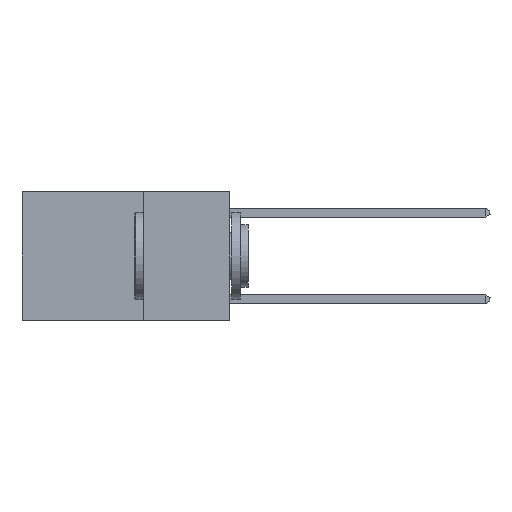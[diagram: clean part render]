
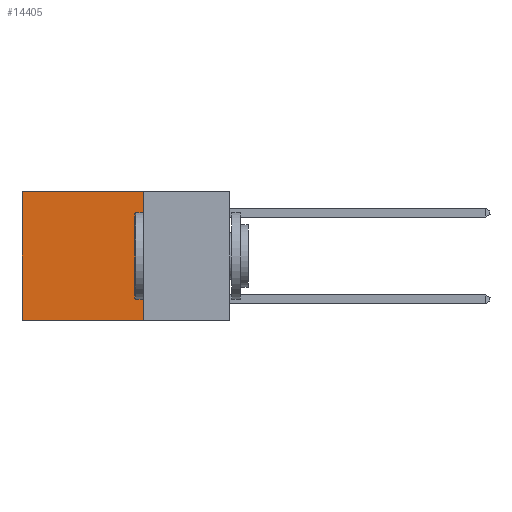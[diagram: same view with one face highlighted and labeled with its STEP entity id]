
A CAD part, left-side view. The second image highlights one B-rep face of the part: STEP entity #14405.
In plain terms, the highlighted planar face has unit normal (-1, 0, 0).
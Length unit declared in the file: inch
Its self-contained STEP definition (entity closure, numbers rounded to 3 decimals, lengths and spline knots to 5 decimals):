
#430 = CARTESIAN_POINT ( 'NONE',  ( 0.2625, 0.25, 0. ) ) ;
#1091 = CARTESIAN_POINT ( 'NONE',  ( 0.2625, 0.25, 0. ) ) ;
#1458 = PLANE ( 'NONE',  #2415 ) ;
#2415 = AXIS2_PLACEMENT_3D ( 'NONE', #7241, #9456, #25208 ) ;
#2458 = ORIENTED_EDGE ( 'NONE', *, *, #23959, .T. ) ;
#2859 = VECTOR ( 'NONE', #14581, 39.37008 ) ;
#3548 = FACE_OUTER_BOUND ( 'NONE', #19269, .T. ) ;
#3640 = DIRECTION ( 'NONE',  ( 0., 0., -1. ) ) ;
#3770 = CARTESIAN_POINT ( 'NONE',  ( 0.2625, 0.6, 0. ) ) ;
#4625 = DIRECTION ( 'NONE',  ( 0., 0., -1. ) ) ;
#4853 = VERTEX_POINT ( 'NONE', #15897 ) ;
#6142 = LINE ( 'NONE', #3770, #8516 ) ;
#7241 = CARTESIAN_POINT ( 'NONE',  ( 0.2625, 0.25, 0. ) ) ;
#8516 = VECTOR ( 'NONE', #3640, 39.37008 ) ;
#8641 = EDGE_CURVE ( 'NONE', #22225, #14238, #16715, .T. ) ;
#9456 = DIRECTION ( 'NONE',  ( 1., 0., 0. ) ) ;
#12428 = EDGE_CURVE ( 'NONE', #19078, #22225, #18815, .T. ) ;
#13991 = CARTESIAN_POINT ( 'NONE',  ( 0.2625, 0.25, -0.37 ) ) ;
#14238 = VERTEX_POINT ( 'NONE', #22727 ) ;
#14405 = ADVANCED_FACE ( 'NONE', ( #3548 ), #1458, .F. ) ;
#14581 = DIRECTION ( 'NONE',  ( 0., 1., 0. ) ) ;
#15897 = CARTESIAN_POINT ( 'NONE',  ( 0.2625, 0.6, 0. ) ) ;
#16577 = VECTOR ( 'NONE', #4625, 39.37008 ) ;
#16595 = DIRECTION ( 'NONE',  ( 0., 1., 0. ) ) ;
#16604 = VECTOR ( 'NONE', #16595, 39.37008 ) ;
#16608 = EDGE_CURVE ( 'NONE', #19078, #4853, #24304, .T. ) ;
#16715 = LINE ( 'NONE', #13991, #16604 ) ;
#17031 = ORIENTED_EDGE ( 'NONE', *, *, #8641, .F. ) ;
#17127 = CARTESIAN_POINT ( 'NONE',  ( 0.2625, 0.25, -0.37 ) ) ;
#17545 = ORIENTED_EDGE ( 'NONE', *, *, #12428, .F. ) ;
#17815 = ORIENTED_EDGE ( 'NONE', *, *, #16608, .T. ) ;
#18815 = LINE ( 'NONE', #1091, #16577 ) ;
#19078 = VERTEX_POINT ( 'NONE', #430 ) ;
#19269 = EDGE_LOOP ( 'NONE', ( #2458, #17031, #17545, #17815 ) ) ;
#20500 = CARTESIAN_POINT ( 'NONE',  ( 0.2625, 0.25, 0. ) ) ;
#22225 = VERTEX_POINT ( 'NONE', #17127 ) ;
#22727 = CARTESIAN_POINT ( 'NONE',  ( 0.2625, 0.6, -0.37 ) ) ;
#23959 = EDGE_CURVE ( 'NONE', #4853, #14238, #6142, .T. ) ;
#24304 = LINE ( 'NONE', #20500, #2859 ) ;
#25208 = DIRECTION ( 'NONE',  ( 0., 0., -1. ) ) ;
